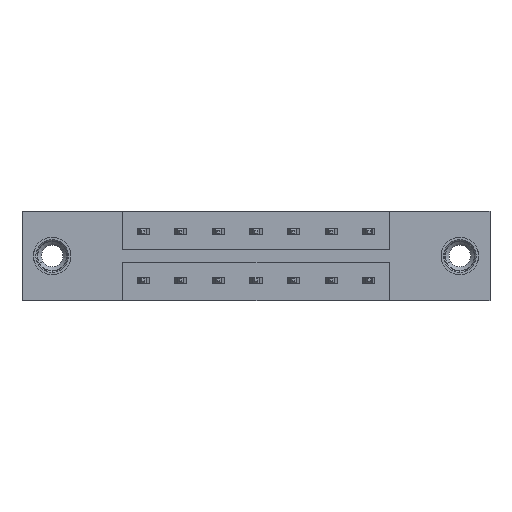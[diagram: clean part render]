
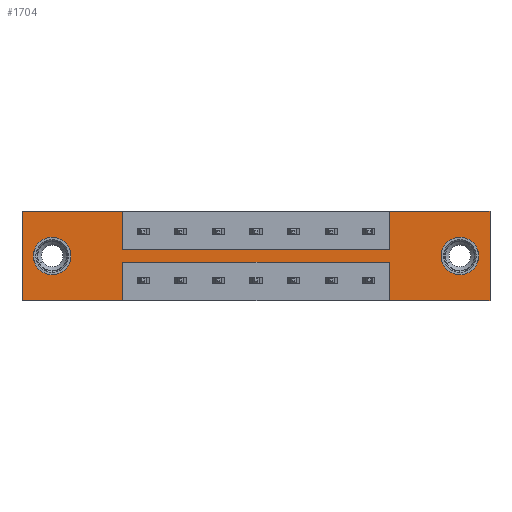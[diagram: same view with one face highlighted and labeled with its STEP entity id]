
A CAD part, front view. The second image highlights one B-rep face of the part: STEP entity #1704.
In plain terms, the highlighted planar face has unit normal (0, -1, 0).
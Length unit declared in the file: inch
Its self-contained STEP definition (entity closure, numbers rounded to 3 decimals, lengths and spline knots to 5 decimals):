
#76 = VERTEX_POINT ( 'NONE', #4168 ) ;
#160 = LINE ( 'NONE', #8924, #2366 ) ;
#208 = AXIS2_PLACEMENT_3D ( 'NONE', #4533, #7792, #5365 ) ;
#224 = ORIENTED_EDGE ( 'NONE', *, *, #7403, .F. ) ;
#245 = DIRECTION ( 'NONE',  ( 0., 0., 1. ) ) ;
#257 = PLANE ( 'NONE',  #5840 ) ;
#284 = VECTOR ( 'NONE', #1515, 39.37008 ) ;
#315 = FACE_BOUND ( 'NONE', #3675, .T. ) ;
#603 = CIRCLE ( 'NONE', #7819, 0.078 ) ;
#660 = DIRECTION ( 'NONE',  ( -1., 0., 0. ) ) ;
#700 = VECTOR ( 'NONE', #3326, 39.37008 ) ;
#853 = CARTESIAN_POINT ( 'NONE',  ( 1.5225, 0., 0. ) ) ;
#895 = EDGE_CURVE ( 'NONE', #5227, #7539, #3608, .T. ) ;
#1046 = CARTESIAN_POINT ( 'NONE',  ( 1.815, 0., -0.107 ) ) ;
#1089 = CARTESIAN_POINT ( 'NONE',  ( 1.94, 0., 0. ) ) ;
#1213 = VECTOR ( 'NONE', #6276, 39.37008 ) ;
#1230 = CARTESIAN_POINT ( 'NONE',  ( 1.94, 0., -0.37 ) ) ;
#1244 = DIRECTION ( 'NONE',  ( 0., 0., 1. ) ) ;
#1515 = DIRECTION ( 'NONE',  ( -1., 0., 0. ) ) ;
#1682 = VECTOR ( 'NONE', #8426, 39.37008 ) ;
#1704 = ADVANCED_FACE ( 'NONE', ( #315, #8928, #5980 ), #257, .T. ) ;
#1792 = VERTEX_POINT ( 'NONE', #8460 ) ;
#1838 = CARTESIAN_POINT ( 'NONE',  ( 0., 0., -0.37 ) ) ;
#1848 = VECTOR ( 'NONE', #7607, 39.37008 ) ;
#1908 = DIRECTION ( 'NONE',  ( 0., 0., -1. ) ) ;
#1912 = EDGE_CURVE ( 'NONE', #7336, #76, #6026, .T. ) ;
#1959 = VECTOR ( 'NONE', #8344, 39.37008 ) ;
#2363 = ORIENTED_EDGE ( 'NONE', *, *, #7622, .F. ) ;
#2366 = VECTOR ( 'NONE', #4784, 39.37008 ) ;
#2589 = LINE ( 'NONE', #7164, #700 ) ;
#2738 = DIRECTION ( 'NONE',  ( 0., 1., 0. ) ) ;
#2942 = CARTESIAN_POINT ( 'NONE',  ( 0.125, 0., -0.107 ) ) ;
#3139 = CIRCLE ( 'NONE', #7116, 0.078 ) ;
#3197 = CARTESIAN_POINT ( 'NONE',  ( 1.815, 0., -0.263 ) ) ;
#3326 = DIRECTION ( 'NONE',  ( 0., 0., 1. ) ) ;
#3425 = DIRECTION ( 'NONE',  ( 0., -1., 0. ) ) ;
#3480 = CARTESIAN_POINT ( 'NONE',  ( 0., 0., -0.37 ) ) ;
#3497 = ORIENTED_EDGE ( 'NONE', *, *, #7275, .T. ) ;
#3566 = LINE ( 'NONE', #5960, #1959 ) ;
#3567 = ORIENTED_EDGE ( 'NONE', *, *, #7745, .T. ) ;
#3608 = LINE ( 'NONE', #9835, #9456 ) ;
#3675 = EDGE_LOOP ( 'NONE', ( #3497, #3567 ) ) ;
#3716 = CARTESIAN_POINT ( 'NONE',  ( 1.5225, 0., -0.2115 ) ) ;
#3779 = EDGE_CURVE ( 'NONE', #1792, #7268, #3566, .T. ) ;
#3791 = VECTOR ( 'NONE', #6261, 39.37008 ) ;
#3816 = CARTESIAN_POINT ( 'NONE',  ( 0.4175, 0., -0.2115 ) ) ;
#3846 = VERTEX_POINT ( 'NONE', #2942 ) ;
#3936 = EDGE_CURVE ( 'NONE', #7539, #6797, #6360, .T. ) ;
#3947 = VERTEX_POINT ( 'NONE', #3197 ) ;
#3948 = ORIENTED_EDGE ( 'NONE', *, *, #5340, .T. ) ;
#4009 = CARTESIAN_POINT ( 'NONE',  ( 0.4175, 0., -0.1585 ) ) ;
#4037 = CARTESIAN_POINT ( 'NONE',  ( 1.94, 0., 0. ) ) ;
#4059 = ORIENTED_EDGE ( 'NONE', *, *, #3779, .F. ) ;
#4168 = CARTESIAN_POINT ( 'NONE',  ( 0.4175, 0., -0.2115 ) ) ;
#4250 = DIRECTION ( 'NONE',  ( 0., 1., 0. ) ) ;
#4413 = CARTESIAN_POINT ( 'NONE',  ( 1.5225, 0., -0.1585 ) ) ;
#4475 = VECTOR ( 'NONE', #660, 39.37008 ) ;
#4533 = CARTESIAN_POINT ( 'NONE',  ( 1.815, 0., -0.185 ) ) ;
#4587 = EDGE_CURVE ( 'NONE', #7719, #7336, #5775, .T. ) ;
#4784 = DIRECTION ( 'NONE',  ( 1., 0., 0. ) ) ;
#5100 = CIRCLE ( 'NONE', #10231, 0.078 ) ;
#5119 = DIRECTION ( 'NONE',  ( 0., 0., -1. ) ) ;
#5186 = VECTOR ( 'NONE', #1244, 39.37008 ) ;
#5227 = VERTEX_POINT ( 'NONE', #7480 ) ;
#5281 = ORIENTED_EDGE ( 'NONE', *, *, #1912, .F. ) ;
#5299 = ORIENTED_EDGE ( 'NONE', *, *, #8276, .F. ) ;
#5340 = EDGE_CURVE ( 'NONE', #3846, #5881, #3139, .T. ) ;
#5365 = DIRECTION ( 'NONE',  ( 0., 0., -1. ) ) ;
#5664 = EDGE_CURVE ( 'NONE', #5881, #3846, #5100, .T. ) ;
#5775 = LINE ( 'NONE', #9612, #6605 ) ;
#5792 = EDGE_CURVE ( 'NONE', #6735, #7719, #8746, .T. ) ;
#5840 = AXIS2_PLACEMENT_3D ( 'NONE', #3480, #3425, #1908 ) ;
#5881 = VERTEX_POINT ( 'NONE', #6887 ) ;
#5960 = CARTESIAN_POINT ( 'NONE',  ( 0., 0., -0.37 ) ) ;
#5980 = FACE_OUTER_BOUND ( 'NONE', #9241, .T. ) ;
#5989 = CARTESIAN_POINT ( 'NONE',  ( 1.5225, 0., -0.1585 ) ) ;
#6016 = ORIENTED_EDGE ( 'NONE', *, *, #7632, .F. ) ;
#6026 = LINE ( 'NONE', #7579, #4475 ) ;
#6167 = ORIENTED_EDGE ( 'NONE', *, *, #3936, .F. ) ;
#6179 = DIRECTION ( 'NONE',  ( 0., 1., 0. ) ) ;
#6261 = DIRECTION ( 'NONE',  ( 1., 0., 0. ) ) ;
#6276 = DIRECTION ( 'NONE',  ( 1., 0., 0. ) ) ;
#6360 = LINE ( 'NONE', #6931, #3791 ) ;
#6605 = VECTOR ( 'NONE', #8790, 39.37008 ) ;
#6632 = ORIENTED_EDGE ( 'NONE', *, *, #7964, .F. ) ;
#6735 = VERTEX_POINT ( 'NONE', #1230 ) ;
#6797 = VERTEX_POINT ( 'NONE', #4413 ) ;
#6880 = LINE ( 'NONE', #3816, #1848 ) ;
#6887 = CARTESIAN_POINT ( 'NONE',  ( 0.125, 0., -0.263 ) ) ;
#6931 = CARTESIAN_POINT ( 'NONE',  ( 0.4175, 0., -0.1585 ) ) ;
#6970 = ORIENTED_EDGE ( 'NONE', *, *, #7965, .F. ) ;
#6997 = VERTEX_POINT ( 'NONE', #4037 ) ;
#7116 = AXIS2_PLACEMENT_3D ( 'NONE', #10119, #6179, #9294 ) ;
#7164 = CARTESIAN_POINT ( 'NONE',  ( 0., 0., 0. ) ) ;
#7268 = VERTEX_POINT ( 'NONE', #1838 ) ;
#7275 = EDGE_CURVE ( 'NONE', #9550, #3947, #603, .T. ) ;
#7336 = VERTEX_POINT ( 'NONE', #3716 ) ;
#7344 = EDGE_LOOP ( 'NONE', ( #3948, #7437 ) ) ;
#7354 = CARTESIAN_POINT ( 'NONE',  ( 1.815, 0., -0.185 ) ) ;
#7398 = CARTESIAN_POINT ( 'NONE',  ( 0., 0., 0. ) ) ;
#7403 = EDGE_CURVE ( 'NONE', #76, #1792, #6880, .T. ) ;
#7437 = ORIENTED_EDGE ( 'NONE', *, *, #5664, .T. ) ;
#7480 = CARTESIAN_POINT ( 'NONE',  ( 0.4175, 0., 0. ) ) ;
#7539 = VERTEX_POINT ( 'NONE', #4009 ) ;
#7542 = LINE ( 'NONE', #5989, #5186 ) ;
#7579 = CARTESIAN_POINT ( 'NONE',  ( 0.4175, 0., -0.2115 ) ) ;
#7607 = DIRECTION ( 'NONE',  ( 0., 0., -1. ) ) ;
#7622 = EDGE_CURVE ( 'NONE', #6997, #6735, #8371, .T. ) ;
#7632 = EDGE_CURVE ( 'NONE', #6797, #8923, #7542, .T. ) ;
#7719 = VERTEX_POINT ( 'NONE', #8989 ) ;
#7745 = EDGE_CURVE ( 'NONE', #3947, #9550, #8500, .T. ) ;
#7778 = CARTESIAN_POINT ( 'NONE',  ( 0., 0., 0. ) ) ;
#7792 = DIRECTION ( 'NONE',  ( 0., 1., 0. ) ) ;
#7819 = AXIS2_PLACEMENT_3D ( 'NONE', #7354, #2738, #8181 ) ;
#7964 = EDGE_CURVE ( 'NONE', #9078, #5227, #160, .T. ) ;
#7965 = EDGE_CURVE ( 'NONE', #7268, #9078, #2589, .T. ) ;
#8181 = DIRECTION ( 'NONE',  ( 0., 0., -1. ) ) ;
#8189 = CARTESIAN_POINT ( 'NONE',  ( 0.125, 0., -0.185 ) ) ;
#8276 = EDGE_CURVE ( 'NONE', #8923, #6997, #10115, .T. ) ;
#8344 = DIRECTION ( 'NONE',  ( -1., 0., 0. ) ) ;
#8345 = ORIENTED_EDGE ( 'NONE', *, *, #4587, .F. ) ;
#8371 = LINE ( 'NONE', #1089, #1682 ) ;
#8426 = DIRECTION ( 'NONE',  ( 0., 0., -1. ) ) ;
#8460 = CARTESIAN_POINT ( 'NONE',  ( 0.4175, 0., -0.37 ) ) ;
#8500 = CIRCLE ( 'NONE', #208, 0.078 ) ;
#8746 = LINE ( 'NONE', #10247, #284 ) ;
#8790 = DIRECTION ( 'NONE',  ( 0., 0., 1. ) ) ;
#8923 = VERTEX_POINT ( 'NONE', #853 ) ;
#8924 = CARTESIAN_POINT ( 'NONE',  ( 0., 0., 0. ) ) ;
#8928 = FACE_BOUND ( 'NONE', #7344, .T. ) ;
#8989 = CARTESIAN_POINT ( 'NONE',  ( 1.5225, 0., -0.37 ) ) ;
#9078 = VERTEX_POINT ( 'NONE', #7398 ) ;
#9241 = EDGE_LOOP ( 'NONE', ( #8345, #9918, #2363, #5299, #6016, #6167, #9942, #6632, #6970, #4059, #224, #5281 ) ) ;
#9294 = DIRECTION ( 'NONE',  ( 0., 0., 1. ) ) ;
#9456 = VECTOR ( 'NONE', #5119, 39.37008 ) ;
#9550 = VERTEX_POINT ( 'NONE', #1046 ) ;
#9612 = CARTESIAN_POINT ( 'NONE',  ( 1.5225, 0., -0.2115 ) ) ;
#9835 = CARTESIAN_POINT ( 'NONE',  ( 0.4175, 0., -0.1585 ) ) ;
#9918 = ORIENTED_EDGE ( 'NONE', *, *, #5792, .F. ) ;
#9942 = ORIENTED_EDGE ( 'NONE', *, *, #895, .F. ) ;
#10115 = LINE ( 'NONE', #7778, #1213 ) ;
#10119 = CARTESIAN_POINT ( 'NONE',  ( 0.125, 0., -0.185 ) ) ;
#10231 = AXIS2_PLACEMENT_3D ( 'NONE', #8189, #4250, #245 ) ;
#10247 = CARTESIAN_POINT ( 'NONE',  ( 0., 0., -0.37 ) ) ;
